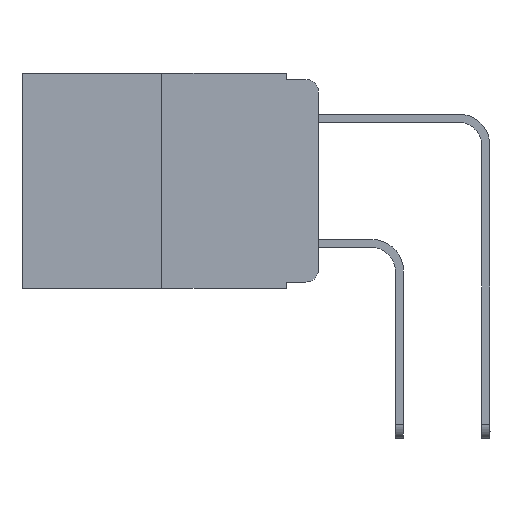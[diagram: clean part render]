
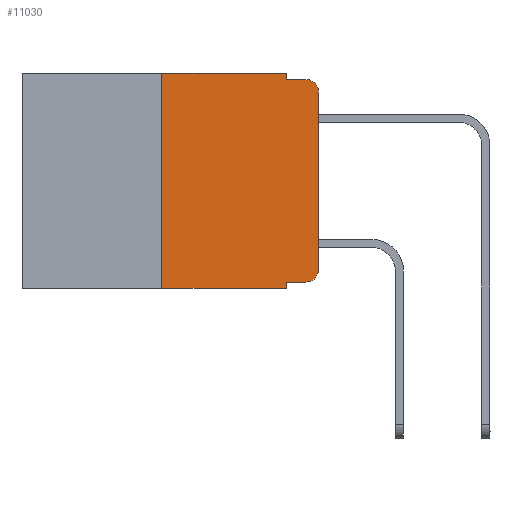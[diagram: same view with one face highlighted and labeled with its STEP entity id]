
A CAD part, left-side view. The second image highlights one B-rep face of the part: STEP entity #11030.
In plain terms, the highlighted planar face has unit normal (-1, 0, 0).
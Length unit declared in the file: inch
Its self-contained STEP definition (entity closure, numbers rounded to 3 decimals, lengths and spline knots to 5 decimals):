
#84 = LINE ( 'NONE', #16614, #1577 ) ;
#240 = DIRECTION ( 'NONE',  ( 1., 0., 0. ) ) ;
#259 = ORIENTED_EDGE ( 'NONE', *, *, #6631, .T. ) ;
#854 = DIRECTION ( 'NONE',  ( 0., 0., -1. ) ) ;
#1577 = VECTOR ( 'NONE', #18195, 39.37008 ) ;
#1677 = CARTESIAN_POINT ( 'NONE',  ( 0., 0.02, -0.01 ) ) ;
#1700 = ORIENTED_EDGE ( 'NONE', *, *, #15002, .F. ) ;
#1963 = CARTESIAN_POINT ( 'NONE',  ( 0., 0.473, 0. ) ) ;
#2118 = CARTESIAN_POINT ( 'NONE',  ( 0., 0.051, -0.333 ) ) ;
#2141 = VECTOR ( 'NONE', #14154, 39.37008 ) ;
#2250 = VERTEX_POINT ( 'NONE', #17630 ) ;
#2305 = EDGE_CURVE ( 'NONE', #15978, #17312, #5905, .T. ) ;
#2494 = VERTEX_POINT ( 'NONE', #6075 ) ;
#2638 = CARTESIAN_POINT ( 'NONE',  ( 0., 0., 0. ) ) ;
#2714 = ORIENTED_EDGE ( 'NONE', *, *, #9771, .T. ) ;
#3315 = ORIENTED_EDGE ( 'NONE', *, *, #13077, .T. ) ;
#3513 = PLANE ( 'NONE',  #15673 ) ;
#3657 = ORIENTED_EDGE ( 'NONE', *, *, #17466, .T. ) ;
#3750 = EDGE_CURVE ( 'NONE', #17312, #5369, #17904, .T. ) ;
#4040 = CARTESIAN_POINT ( 'NONE',  ( 0., 0.02, -0.313 ) ) ;
#4147 = EDGE_CURVE ( 'NONE', #5369, #15021, #6057, .T. ) ;
#4585 = VECTOR ( 'NONE', #12812, 39.37008 ) ;
#5369 = VERTEX_POINT ( 'NONE', #8260 ) ;
#5579 = DIRECTION ( 'NONE',  ( 0., 0., -1. ) ) ;
#5905 = LINE ( 'NONE', #6700, #13593 ) ;
#6057 = LINE ( 'NONE', #14247, #11592 ) ;
#6075 = CARTESIAN_POINT ( 'NONE',  ( 0., 0.051, -0.333 ) ) ;
#6355 = CARTESIAN_POINT ( 'NONE',  ( 0., 0.25, 0. ) ) ;
#6631 = EDGE_CURVE ( 'NONE', #19880, #15021, #9111, .T. ) ;
#6700 = CARTESIAN_POINT ( 'NONE',  ( 0., 0.473, 0. ) ) ;
#6704 = FACE_OUTER_BOUND ( 'NONE', #6798, .T. ) ;
#6742 = VERTEX_POINT ( 'NONE', #19286 ) ;
#6798 = EDGE_LOOP ( 'NONE', ( #15558, #259, #10360, #14791, #12399, #1700, #3315, #11912, #2714, #3657 ) ) ;
#7037 = VERTEX_POINT ( 'NONE', #14222 ) ;
#7731 = VECTOR ( 'NONE', #5579, 39.37008 ) ;
#8122 = DIRECTION ( 'NONE',  ( 0., -1., 0. ) ) ;
#8240 = CARTESIAN_POINT ( 'NONE',  ( 0., 0.051, 0. ) ) ;
#8260 = CARTESIAN_POINT ( 'NONE',  ( 0., 0.051, -0.01 ) ) ;
#8299 = DIRECTION ( 'NONE',  ( 0., -1., 0. ) ) ;
#8439 = DIRECTION ( 'NONE',  ( 0., 0., -1. ) ) ;
#8460 = DIRECTION ( 'NONE',  ( 0., 0., -1. ) ) ;
#8855 = VERTEX_POINT ( 'NONE', #14975 ) ;
#9111 = CIRCLE ( 'NONE', #18395, 0.02 ) ;
#9771 = EDGE_CURVE ( 'NONE', #2494, #2250, #19100, .T. ) ;
#9895 = VECTOR ( 'NONE', #8460, 39.37008 ) ;
#10360 = ORIENTED_EDGE ( 'NONE', *, *, #4147, .F. ) ;
#10802 = EDGE_CURVE ( 'NONE', #7037, #19880, #16887, .T. ) ;
#11030 = ADVANCED_FACE ( 'NONE', ( #6704 ), #3513, .F. ) ;
#11317 = CARTESIAN_POINT ( 'NONE',  ( 0., 0.051, 0. ) ) ;
#11592 = VECTOR ( 'NONE', #8122, 39.37008 ) ;
#11833 = CARTESIAN_POINT ( 'NONE',  ( 0., 0.051, 0. ) ) ;
#11912 = ORIENTED_EDGE ( 'NONE', *, *, #18166, .F. ) ;
#12399 = ORIENTED_EDGE ( 'NONE', *, *, #2305, .F. ) ;
#12812 = DIRECTION ( 'NONE',  ( 0., -1., 0. ) ) ;
#12990 = LINE ( 'NONE', #11833, #7731 ) ;
#13077 = EDGE_CURVE ( 'NONE', #8855, #6742, #84, .T. ) ;
#13149 = CARTESIAN_POINT ( 'NONE',  ( 0., 0.02, -0.03 ) ) ;
#13154 = CARTESIAN_POINT ( 'NONE',  ( 0., 0.25, 0. ) ) ;
#13593 = VECTOR ( 'NONE', #8299, 39.37008 ) ;
#14154 = DIRECTION ( 'NONE',  ( 0., 0., 1. ) ) ;
#14222 = CARTESIAN_POINT ( 'NONE',  ( 0., 0., -0.313 ) ) ;
#14247 = CARTESIAN_POINT ( 'NONE',  ( 0., 0.051, -0.01 ) ) ;
#14791 = ORIENTED_EDGE ( 'NONE', *, *, #3750, .F. ) ;
#14975 = CARTESIAN_POINT ( 'NONE',  ( 0., 0.25, -0.343 ) ) ;
#15002 = EDGE_CURVE ( 'NONE', #8855, #15978, #17151, .T. ) ;
#15021 = VERTEX_POINT ( 'NONE', #1677 ) ;
#15236 = AXIS2_PLACEMENT_3D ( 'NONE', #4040, #19604, #854 ) ;
#15558 = ORIENTED_EDGE ( 'NONE', *, *, #10802, .T. ) ;
#15673 = AXIS2_PLACEMENT_3D ( 'NONE', #1963, #240, #17160 ) ;
#15978 = VERTEX_POINT ( 'NONE', #13154 ) ;
#16485 = DIRECTION ( 'NONE',  ( -1., 0., 0. ) ) ;
#16614 = CARTESIAN_POINT ( 'NONE',  ( 0., 0.473, -0.343 ) ) ;
#16887 = LINE ( 'NONE', #2638, #18822 ) ;
#17151 = LINE ( 'NONE', #6355, #2141 ) ;
#17160 = DIRECTION ( 'NONE',  ( 0., 0., -1. ) ) ;
#17312 = VERTEX_POINT ( 'NONE', #11317 ) ;
#17466 = EDGE_CURVE ( 'NONE', #2250, #7037, #17667, .T. ) ;
#17630 = CARTESIAN_POINT ( 'NONE',  ( 0., 0.02, -0.333 ) ) ;
#17667 = CIRCLE ( 'NONE', #15236, 0.02 ) ;
#17904 = LINE ( 'NONE', #8240, #9895 ) ;
#18166 = EDGE_CURVE ( 'NONE', #2494, #6742, #12990, .T. ) ;
#18195 = DIRECTION ( 'NONE',  ( 0., -1., 0. ) ) ;
#18395 = AXIS2_PLACEMENT_3D ( 'NONE', #13149, #16485, #8439 ) ;
#18822 = VECTOR ( 'NONE', #19462, 39.37008 ) ;
#19100 = LINE ( 'NONE', #2118, #4585 ) ;
#19112 = CARTESIAN_POINT ( 'NONE',  ( 0., 0., -0.03 ) ) ;
#19286 = CARTESIAN_POINT ( 'NONE',  ( 0., 0.051, -0.343 ) ) ;
#19462 = DIRECTION ( 'NONE',  ( 0., 0., 1. ) ) ;
#19604 = DIRECTION ( 'NONE',  ( -1., 0., 0. ) ) ;
#19880 = VERTEX_POINT ( 'NONE', #19112 ) ;
